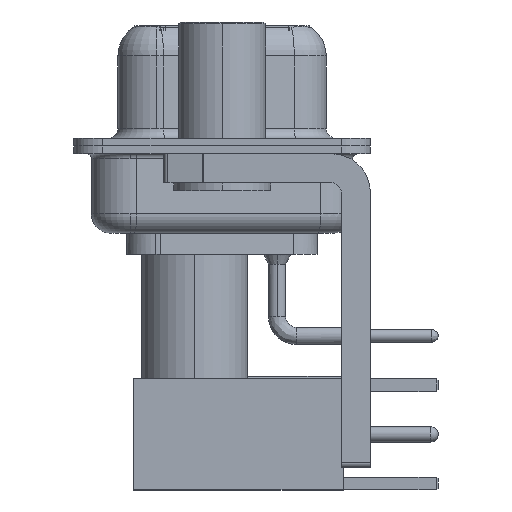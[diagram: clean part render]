
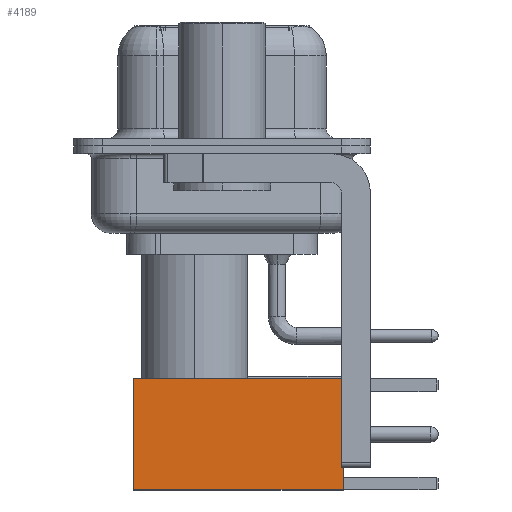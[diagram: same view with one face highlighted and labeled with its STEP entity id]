
A CAD part, left-side view. The second image highlights one B-rep face of the part: STEP entity #4189.
In plain terms, the highlighted face is planar.
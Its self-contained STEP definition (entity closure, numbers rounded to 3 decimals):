
#627 = FACE_OUTER_BOUND ( 'NONE', #32983, .T. ) ;
#4189 = ADVANCED_FACE ( 'NONE', ( #627 ), #18897, .T. ) ;
#4530 = DIRECTION ( 'NONE',  ( 0., 0., -1. ) ) ;
#9765 = CARTESIAN_POINT ( 'NONE',  ( 2.875, 2.875, 0. ) ) ;
#10196 = CARTESIAN_POINT ( 'NONE',  ( 0., 2.875, 10.82 ) ) ;
#11925 = ORIENTED_EDGE ( 'NONE', *, *, #26647, .T. ) ;
#12500 = DIRECTION ( 'NONE',  ( 0., 1., 0. ) ) ;
#13640 = LINE ( 'NONE', #28404, #37766 ) ;
#14360 = EDGE_CURVE ( 'NONE', #31237, #20836, #25193, .T. ) ;
#15019 = VERTEX_POINT ( 'NONE', #26376 ) ;
#17034 = CARTESIAN_POINT ( 'NONE',  ( -2.875, 2.875, 10.82 ) ) ;
#18897 = PLANE ( 'NONE',  #36715 ) ;
#20836 = VERTEX_POINT ( 'NONE', #17034 ) ;
#21631 = DIRECTION ( 'NONE',  ( 0., 0., 1. ) ) ;
#22045 = CARTESIAN_POINT ( 'NONE',  ( -2.875, 2.875, 0. ) ) ;
#22532 = CARTESIAN_POINT ( 'NONE',  ( 0., 2.875, 0. ) ) ;
#22652 = DIRECTION ( 'NONE',  ( -1., 0., 0. ) ) ;
#24879 = ORIENTED_EDGE ( 'NONE', *, *, #25124, .T. ) ;
#25124 = EDGE_CURVE ( 'NONE', #28850, #15019, #27780, .T. ) ;
#25193 = LINE ( 'NONE', #10196, #26082 ) ;
#25528 = VECTOR ( 'NONE', #4530, 1000. ) ;
#25670 = ORIENTED_EDGE ( 'NONE', *, *, #29287, .F. ) ;
#26082 = VECTOR ( 'NONE', #22652, 1000. ) ;
#26376 = CARTESIAN_POINT ( 'NONE',  ( -2.875, 2.875, 0. ) ) ;
#26647 = EDGE_CURVE ( 'NONE', #31237, #28850, #13640, .T. ) ;
#27780 = LINE ( 'NONE', #22532, #29697 ) ;
#28404 = CARTESIAN_POINT ( 'NONE',  ( 2.875, 2.875, 0. ) ) ;
#28850 = VERTEX_POINT ( 'NONE', #31275 ) ;
#29189 = CARTESIAN_POINT ( 'NONE',  ( 2.875, 2.875, 10.82 ) ) ;
#29287 = EDGE_CURVE ( 'NONE', #20836, #15019, #31187, .T. ) ;
#29697 = VECTOR ( 'NONE', #31457, 1000. ) ;
#31187 = LINE ( 'NONE', #22045, #25528 ) ;
#31237 = VERTEX_POINT ( 'NONE', #29189 ) ;
#31275 = CARTESIAN_POINT ( 'NONE',  ( 2.875, 2.875, 0. ) ) ;
#31457 = DIRECTION ( 'NONE',  ( -1., 0., 0. ) ) ;
#32983 = EDGE_LOOP ( 'NONE', ( #11925, #24879, #25670, #36361 ) ) ;
#34238 = DIRECTION ( 'NONE',  ( 0., 0., -1. ) ) ;
#36361 = ORIENTED_EDGE ( 'NONE', *, *, #14360, .F. ) ;
#36715 = AXIS2_PLACEMENT_3D ( 'NONE', #9765, #12500, #21631 ) ;
#37766 = VECTOR ( 'NONE', #34238, 1000. ) ;
